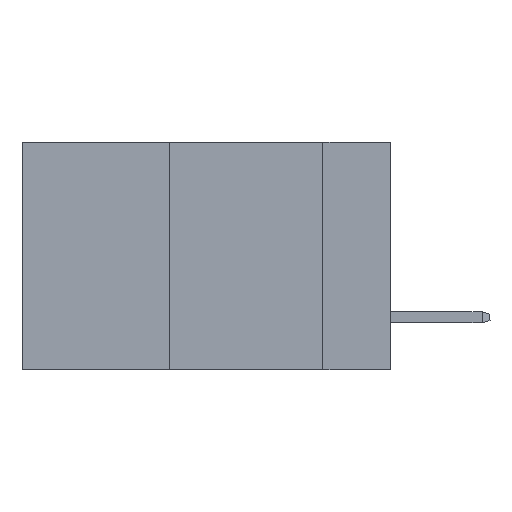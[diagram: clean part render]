
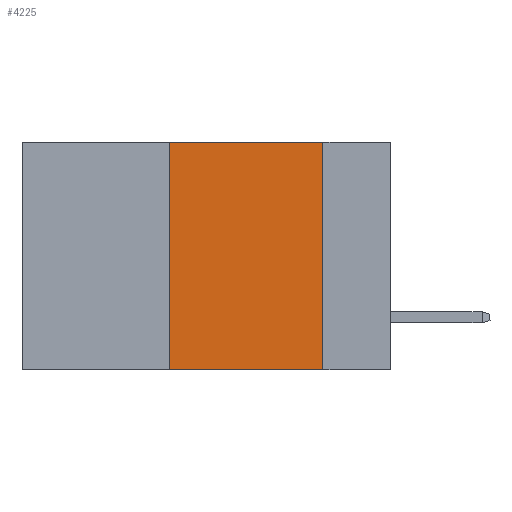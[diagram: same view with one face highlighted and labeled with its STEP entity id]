
A CAD part, left-side view. The second image highlights one B-rep face of the part: STEP entity #4225.
In plain terms, the highlighted planar face has unit normal (-1, 0, 0).
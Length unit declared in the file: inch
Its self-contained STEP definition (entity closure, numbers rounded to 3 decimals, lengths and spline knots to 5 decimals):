
#18 = CARTESIAN_POINT ( 'NONE',  ( 0., 0.6, -0.37 ) ) ;
#104 = VERTEX_POINT ( 'NONE', #2985 ) ;
#225 = CARTESIAN_POINT ( 'NONE',  ( 0., 0.36, 0. ) ) ;
#500 = VECTOR ( 'NONE', #967, 39.37008 ) ;
#550 = CARTESIAN_POINT ( 'NONE',  ( 0., 0.11, 0. ) ) ;
#967 = DIRECTION ( 'NONE',  ( 0., -1., 0. ) ) ;
#999 = CARTESIAN_POINT ( 'NONE',  ( 0., 0.36, 0. ) ) ;
#1654 = EDGE_LOOP ( 'NONE', ( #3268, #2703, #3591, #4971 ) ) ;
#1859 = VERTEX_POINT ( 'NONE', #550 ) ;
#2190 = PLANE ( 'NONE',  #3136 ) ;
#2228 = LINE ( 'NONE', #4563, #2663 ) ;
#2663 = VECTOR ( 'NONE', #5390, 39.37008 ) ;
#2703 = ORIENTED_EDGE ( 'NONE', *, *, #4950, .F. ) ;
#2890 = DIRECTION ( 'NONE',  ( 0., 0., -1. ) ) ;
#2985 = CARTESIAN_POINT ( 'NONE',  ( 0., 0.36, -0.37 ) ) ;
#3136 = AXIS2_PLACEMENT_3D ( 'NONE', #3614, #7043, #2890 ) ;
#3268 = ORIENTED_EDGE ( 'NONE', *, *, #3932, .F. ) ;
#3591 = ORIENTED_EDGE ( 'NONE', *, *, #7995, .F. ) ;
#3592 = EDGE_CURVE ( 'NONE', #104, #6395, #4489, .T. ) ;
#3614 = CARTESIAN_POINT ( 'NONE',  ( 0., 0.6, 0. ) ) ;
#3932 = EDGE_CURVE ( 'NONE', #1859, #6395, #2228, .T. ) ;
#3947 = VECTOR ( 'NONE', #4169, 39.37008 ) ;
#4169 = DIRECTION ( 'NONE',  ( 0., -1., 0. ) ) ;
#4225 = ADVANCED_FACE ( 'NONE', ( #7427 ), #2190, .F. ) ;
#4326 = VECTOR ( 'NONE', #5872, 39.37008 ) ;
#4489 = LINE ( 'NONE', #18, #3947 ) ;
#4563 = CARTESIAN_POINT ( 'NONE',  ( 0., 0.11, 0. ) ) ;
#4950 = EDGE_CURVE ( 'NONE', #8504, #1859, #5689, .T. ) ;
#4971 = ORIENTED_EDGE ( 'NONE', *, *, #3592, .T. ) ;
#5390 = DIRECTION ( 'NONE',  ( 0., 0., -1. ) ) ;
#5689 = LINE ( 'NONE', #5779, #500 ) ;
#5779 = CARTESIAN_POINT ( 'NONE',  ( 0., 0.6, 0. ) ) ;
#5872 = DIRECTION ( 'NONE',  ( 0., 0., 1. ) ) ;
#6395 = VERTEX_POINT ( 'NONE', #6600 ) ;
#6600 = CARTESIAN_POINT ( 'NONE',  ( 0., 0.11, -0.37 ) ) ;
#6740 = LINE ( 'NONE', #999, #4326 ) ;
#7043 = DIRECTION ( 'NONE',  ( 1., 0., 0. ) ) ;
#7427 = FACE_OUTER_BOUND ( 'NONE', #1654, .T. ) ;
#7995 = EDGE_CURVE ( 'NONE', #104, #8504, #6740, .T. ) ;
#8504 = VERTEX_POINT ( 'NONE', #225 ) ;
